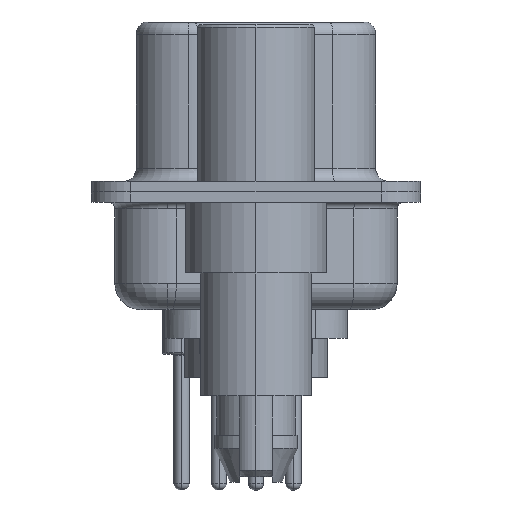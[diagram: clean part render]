
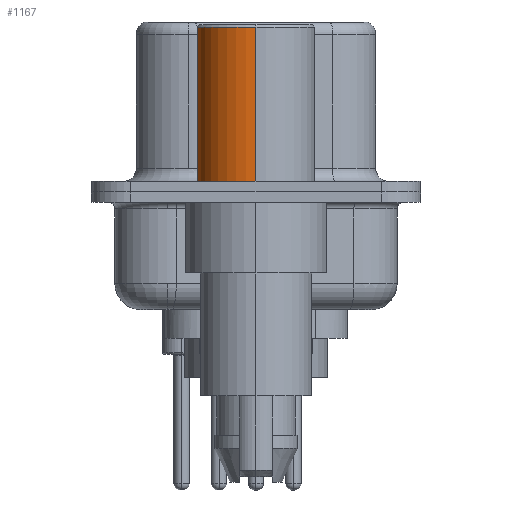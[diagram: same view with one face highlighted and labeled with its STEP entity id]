
A CAD part, left-side view. The second image highlights one B-rep face of the part: STEP entity #1167.
In plain terms, the highlighted cylindrical face has radius 2.25 mm (diameter 4.5 mm), a partial arc.
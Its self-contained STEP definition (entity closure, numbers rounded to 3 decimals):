
#352 = ORIENTED_EDGE ( 'NONE', *, *, #7024, .T. ) ;
#1167 = ADVANCED_FACE ( 'NONE', ( #10856 ), #16174, .T. ) ;
#1561 = EDGE_CURVE ( 'NONE', #11557, #12268, #6024, .T. ) ;
#2469 = ORIENTED_EDGE ( 'NONE', *, *, #6757, .T. ) ;
#2941 = CARTESIAN_POINT ( 'NONE',  ( -2.25, 0., 0.4 ) ) ;
#3521 = CARTESIAN_POINT ( 'NONE',  ( 0., 0., 0.4 ) ) ;
#3805 = EDGE_CURVE ( 'NONE', #15534, #11557, #9243, .T. ) ;
#4200 = DIRECTION ( 'NONE',  ( 0., 0., 1. ) ) ;
#5936 = DIRECTION ( 'NONE',  ( 1., 0., 0. ) ) ;
#6024 = CIRCLE ( 'NONE', #18587, 2.25 ) ;
#6453 = DIRECTION ( 'NONE',  ( 0., 0., 1. ) ) ;
#6625 = DIRECTION ( 'NONE',  ( 0., 0., 1. ) ) ;
#6757 = EDGE_CURVE ( 'NONE', #12225, #12268, #11397, .T. ) ;
#7024 = EDGE_CURVE ( 'NONE', #15534, #12225, #18487, .T. ) ;
#8119 = CARTESIAN_POINT ( 'NONE',  ( 0., 0., 0.581 ) ) ;
#9045 = CARTESIAN_POINT ( 'NONE',  ( 0., 0., 6.3 ) ) ;
#9243 = LINE ( 'NONE', #16219, #16623 ) ;
#10670 = DIRECTION ( 'NONE',  ( 1., 0., 0. ) ) ;
#10703 = EDGE_LOOP ( 'NONE', ( #352, #2469, #18504, #20191 ) ) ;
#10856 = FACE_OUTER_BOUND ( 'NONE', #10703, .T. ) ;
#11397 = LINE ( 'NONE', #15546, #13459 ) ;
#11557 = VERTEX_POINT ( 'NONE', #17063 ) ;
#12168 = CARTESIAN_POINT ( 'NONE',  ( 2.25, 0., 0.4 ) ) ;
#12225 = VERTEX_POINT ( 'NONE', #2941 ) ;
#12268 = VERTEX_POINT ( 'NONE', #16363 ) ;
#12297 = DIRECTION ( 'NONE',  ( 0., 0., 1. ) ) ;
#13458 = AXIS2_PLACEMENT_3D ( 'NONE', #8119, #6625, #19477 ) ;
#13459 = VECTOR ( 'NONE', #17050, 1000. ) ;
#13690 = AXIS2_PLACEMENT_3D ( 'NONE', #3521, #12297, #5936 ) ;
#15534 = VERTEX_POINT ( 'NONE', #12168 ) ;
#15546 = CARTESIAN_POINT ( 'NONE',  ( -2.25, 0., 0.581 ) ) ;
#16174 = CYLINDRICAL_SURFACE ( 'NONE', #13458, 2.25 ) ;
#16219 = CARTESIAN_POINT ( 'NONE',  ( 2.25, 0., 0.581 ) ) ;
#16363 = CARTESIAN_POINT ( 'NONE',  ( -2.25, 0., 6.3 ) ) ;
#16623 = VECTOR ( 'NONE', #6453, 1000. ) ;
#17050 = DIRECTION ( 'NONE',  ( 0., 0., 1. ) ) ;
#17063 = CARTESIAN_POINT ( 'NONE',  ( 2.25, 0., 6.3 ) ) ;
#18487 = CIRCLE ( 'NONE', #13690, 2.25 ) ;
#18504 = ORIENTED_EDGE ( 'NONE', *, *, #1561, .F. ) ;
#18587 = AXIS2_PLACEMENT_3D ( 'NONE', #9045, #4200, #10670 ) ;
#19477 = DIRECTION ( 'NONE',  ( 1., 0., 0. ) ) ;
#20191 = ORIENTED_EDGE ( 'NONE', *, *, #3805, .F. ) ;
